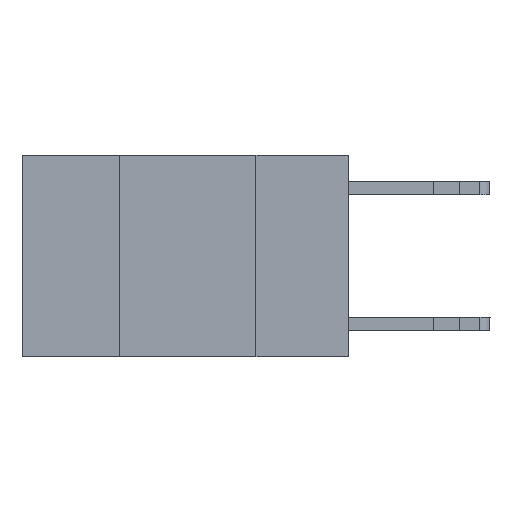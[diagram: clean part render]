
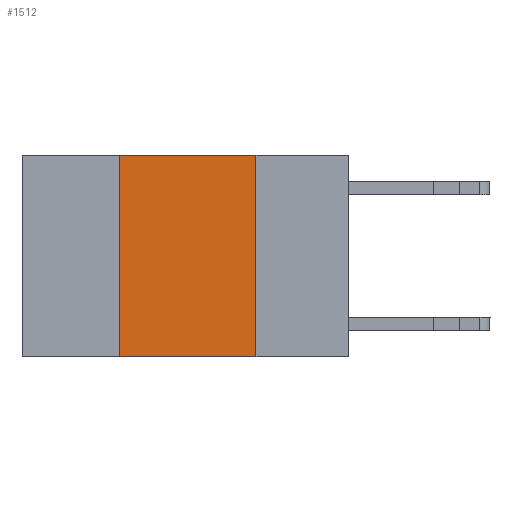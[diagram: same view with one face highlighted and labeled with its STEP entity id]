
A CAD part, left-side view. The second image highlights one B-rep face of the part: STEP entity #1512.
In plain terms, the highlighted planar face has unit normal (-1, 0, 0).
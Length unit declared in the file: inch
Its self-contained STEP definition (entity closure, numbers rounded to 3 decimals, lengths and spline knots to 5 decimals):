
#192 = LINE ( 'NONE', #6682, #8645 ) ;
#640 = PLANE ( 'NONE',  #7743 ) ;
#793 = CARTESIAN_POINT ( 'NONE',  ( 0., 0.17, -0.37 ) ) ;
#1512 = ADVANCED_FACE ( 'NONE', ( #10050 ), #640, .F. ) ;
#2178 = CARTESIAN_POINT ( 'NONE',  ( 0., 0.17, 0. ) ) ;
#2261 = DIRECTION ( 'NONE',  ( 1., 0., 0. ) ) ;
#4023 = VECTOR ( 'NONE', #18743, 39.37008 ) ;
#4122 = EDGE_CURVE ( 'NONE', #5143, #6319, #8478, .T. ) ;
#4284 = VECTOR ( 'NONE', #8599, 39.37008 ) ;
#4588 = CARTESIAN_POINT ( 'NONE',  ( 0., 0.6, 0. ) ) ;
#5092 = ORIENTED_EDGE ( 'NONE', *, *, #17786, .T. ) ;
#5143 = VERTEX_POINT ( 'NONE', #12823 ) ;
#5789 = DIRECTION ( 'NONE',  ( 0., 0., 1. ) ) ;
#6319 = VERTEX_POINT ( 'NONE', #793 ) ;
#6682 = CARTESIAN_POINT ( 'NONE',  ( 0., 0.6, -0.37 ) ) ;
#7743 = AXIS2_PLACEMENT_3D ( 'NONE', #10131, #2261, #13296 ) ;
#7844 = VECTOR ( 'NONE', #5789, 39.37008 ) ;
#8370 = VERTEX_POINT ( 'NONE', #13722 ) ;
#8478 = LINE ( 'NONE', #2178, #4284 ) ;
#8599 = DIRECTION ( 'NONE',  ( 0., 0., -1. ) ) ;
#8645 = VECTOR ( 'NONE', #14618, 39.37008 ) ;
#9882 = ORIENTED_EDGE ( 'NONE', *, *, #4122, .F. ) ;
#10050 = FACE_OUTER_BOUND ( 'NONE', #12096, .T. ) ;
#10131 = CARTESIAN_POINT ( 'NONE',  ( 0., 0.6, 0. ) ) ;
#10204 = EDGE_CURVE ( 'NONE', #8370, #17060, #15746, .T. ) ;
#12096 = EDGE_LOOP ( 'NONE', ( #9882, #20169, #15066, #5092 ) ) ;
#12823 = CARTESIAN_POINT ( 'NONE',  ( 0., 0.17, 0. ) ) ;
#12865 = EDGE_CURVE ( 'NONE', #17060, #5143, #16590, .T. ) ;
#13296 = DIRECTION ( 'NONE',  ( 0., 0., -1. ) ) ;
#13722 = CARTESIAN_POINT ( 'NONE',  ( 0., 0.42, -0.37 ) ) ;
#14441 = CARTESIAN_POINT ( 'NONE',  ( 0., 0.42, 0. ) ) ;
#14618 = DIRECTION ( 'NONE',  ( 0., -1., 0. ) ) ;
#15066 = ORIENTED_EDGE ( 'NONE', *, *, #10204, .F. ) ;
#15746 = LINE ( 'NONE', #16814, #7844 ) ;
#16590 = LINE ( 'NONE', #4588, #4023 ) ;
#16814 = CARTESIAN_POINT ( 'NONE',  ( 0., 0.42, 0. ) ) ;
#17060 = VERTEX_POINT ( 'NONE', #14441 ) ;
#17786 = EDGE_CURVE ( 'NONE', #8370, #6319, #192, .T. ) ;
#18743 = DIRECTION ( 'NONE',  ( 0., -1., 0. ) ) ;
#20169 = ORIENTED_EDGE ( 'NONE', *, *, #12865, .F. ) ;
